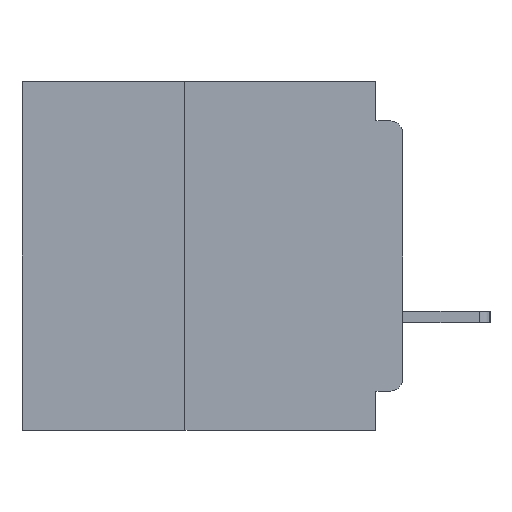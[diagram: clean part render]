
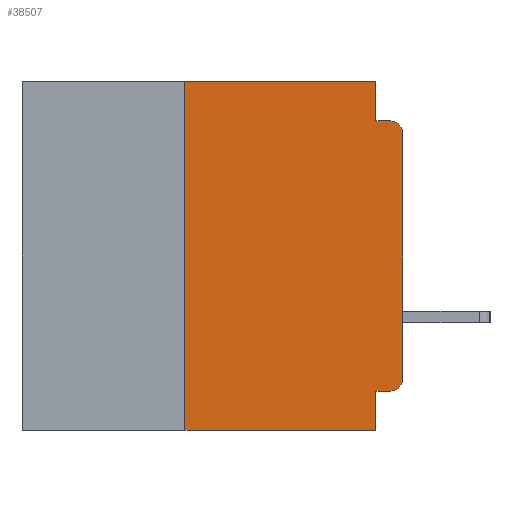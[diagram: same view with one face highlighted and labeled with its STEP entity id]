
A CAD part, left-side view. The second image highlights one B-rep face of the part: STEP entity #38507.
In plain terms, the highlighted planar face has unit normal (-1, 0, 0).
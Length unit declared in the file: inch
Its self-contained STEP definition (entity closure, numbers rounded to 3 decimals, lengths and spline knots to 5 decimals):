
#300 = EDGE_CURVE ( 'NONE', #31197, #36646, #64889, .T. ) ;
#389 = CARTESIAN_POINT ( 'NONE',  ( 0., 0.031, -0.355 ) ) ;
#638 = CARTESIAN_POINT ( 'NONE',  ( 0., 0., -0.06 ) ) ;
#1418 = ORIENTED_EDGE ( 'NONE', *, *, #44566, .F. ) ;
#1502 = DIRECTION ( 'NONE',  ( 0., 0., -1. ) ) ;
#1721 = AXIS2_PLACEMENT_3D ( 'NONE', #28137, #63955, #33288 ) ;
#1724 = EDGE_CURVE ( 'NONE', #13966, #51907, #29463, .T. ) ;
#1972 = CARTESIAN_POINT ( 'NONE',  ( 0., 0.437, 0. ) ) ;
#2990 = VERTEX_POINT ( 'NONE', #50784 ) ;
#3612 = VECTOR ( 'NONE', #39474, 39.37008 ) ;
#4235 = VERTEX_POINT ( 'NONE', #389 ) ;
#4448 = VECTOR ( 'NONE', #34540, 39.37008 ) ;
#4666 = LINE ( 'NONE', #46689, #44174 ) ;
#4717 = CARTESIAN_POINT ( 'NONE',  ( 0., 0.015, -0.045 ) ) ;
#6068 = ORIENTED_EDGE ( 'NONE', *, *, #1724, .T. ) ;
#6707 = LINE ( 'NONE', #27226, #58166 ) ;
#7853 = DIRECTION ( 'NONE',  ( 0., 0., -1. ) ) ;
#7986 = DIRECTION ( 'NONE',  ( -1., 0., 0. ) ) ;
#8141 = CARTESIAN_POINT ( 'NONE',  ( 0., 0.015, -0.06 ) ) ;
#8779 = EDGE_CURVE ( 'NONE', #31197, #39719, #44422, .T. ) ;
#9696 = CARTESIAN_POINT ( 'NONE',  ( 0., 0.437, 0. ) ) ;
#10513 = CIRCLE ( 'NONE', #1721, 0.015 ) ;
#12424 = EDGE_CURVE ( 'NONE', #45989, #31343, #10513, .T. ) ;
#13966 = VERTEX_POINT ( 'NONE', #638 ) ;
#14341 = ORIENTED_EDGE ( 'NONE', *, *, #63527, .F. ) ;
#16952 = VECTOR ( 'NONE', #34377, 39.37008 ) ;
#17418 = LINE ( 'NONE', #18843, #3612 ) ;
#18843 = CARTESIAN_POINT ( 'NONE',  ( 0., 0., -0.355 ) ) ;
#19035 = VECTOR ( 'NONE', #40504, 39.37008 ) ;
#20340 = EDGE_CURVE ( 'NONE', #31343, #13966, #59463, .T. ) ;
#21923 = FACE_OUTER_BOUND ( 'NONE', #22598, .T. ) ;
#22155 = ORIENTED_EDGE ( 'NONE', *, *, #12424, .T. ) ;
#22598 = EDGE_LOOP ( 'NONE', ( #47404, #6068, #56346, #14341, #60851, #65360, #43607, #38839, #1418, #22155 ) ) ;
#22989 = DIRECTION ( 'NONE',  ( 1., 0., 0. ) ) ;
#24036 = VECTOR ( 'NONE', #61606, 39.37008 ) ;
#24302 = EDGE_CURVE ( 'NONE', #36646, #2990, #32620, .T. ) ;
#26323 = CARTESIAN_POINT ( 'NONE',  ( 0., 0.015, -0.355 ) ) ;
#27226 = CARTESIAN_POINT ( 'NONE',  ( 0., 0.031, -0.4 ) ) ;
#28137 = CARTESIAN_POINT ( 'NONE',  ( 0., 0.015, -0.34 ) ) ;
#28972 = CARTESIAN_POINT ( 'NONE',  ( 0., 0.031, -0.4 ) ) ;
#29415 = CARTESIAN_POINT ( 'NONE',  ( 0., 0., -0.34 ) ) ;
#29463 = CIRCLE ( 'NONE', #58442, 0.015 ) ;
#30747 = VECTOR ( 'NONE', #58452, 39.37008 ) ;
#31197 = VERTEX_POINT ( 'NONE', #63880 ) ;
#31343 = VERTEX_POINT ( 'NONE', #29415 ) ;
#32190 = CARTESIAN_POINT ( 'NONE',  ( 0., 0.25, 0. ) ) ;
#32620 = LINE ( 'NONE', #9696, #19035 ) ;
#33288 = DIRECTION ( 'NONE',  ( 0., 0., -1. ) ) ;
#34369 = EDGE_CURVE ( 'NONE', #4235, #39719, #6707, .T. ) ;
#34377 = DIRECTION ( 'NONE',  ( 0., 0., 1. ) ) ;
#34540 = DIRECTION ( 'NONE',  ( 0., 0., -1. ) ) ;
#36646 = VERTEX_POINT ( 'NONE', #32190 ) ;
#38507 = ADVANCED_FACE ( 'NONE', ( #21923 ), #63750, .F. ) ;
#38839 = ORIENTED_EDGE ( 'NONE', *, *, #34369, .F. ) ;
#39474 = DIRECTION ( 'NONE',  ( 0., 1., 0. ) ) ;
#39719 = VERTEX_POINT ( 'NONE', #28972 ) ;
#39935 = VERTEX_POINT ( 'NONE', #56120 ) ;
#40504 = DIRECTION ( 'NONE',  ( 0., -1., 0. ) ) ;
#43607 = ORIENTED_EDGE ( 'NONE', *, *, #8779, .T. ) ;
#44174 = VECTOR ( 'NONE', #51844, 39.37008 ) ;
#44215 = AXIS2_PLACEMENT_3D ( 'NONE', #1972, #22989, #58860 ) ;
#44422 = LINE ( 'NONE', #48177, #30747 ) ;
#44566 = EDGE_CURVE ( 'NONE', #45989, #4235, #17418, .T. ) ;
#45989 = VERTEX_POINT ( 'NONE', #26323 ) ;
#46689 = CARTESIAN_POINT ( 'NONE',  ( 0., 0., -0.045 ) ) ;
#47404 = ORIENTED_EDGE ( 'NONE', *, *, #20340, .T. ) ;
#48177 = CARTESIAN_POINT ( 'NONE',  ( 0., 0.437, -0.4 ) ) ;
#49900 = EDGE_CURVE ( 'NONE', #39935, #51907, #4666, .T. ) ;
#50784 = CARTESIAN_POINT ( 'NONE',  ( 0., 0.031, 0. ) ) ;
#51844 = DIRECTION ( 'NONE',  ( 0., -1., 0. ) ) ;
#51907 = VERTEX_POINT ( 'NONE', #4717 ) ;
#56120 = CARTESIAN_POINT ( 'NONE',  ( 0., 0.031, -0.045 ) ) ;
#56346 = ORIENTED_EDGE ( 'NONE', *, *, #49900, .F. ) ;
#58166 = VECTOR ( 'NONE', #1502, 39.37008 ) ;
#58442 = AXIS2_PLACEMENT_3D ( 'NONE', #8141, #7986, #7853 ) ;
#58452 = DIRECTION ( 'NONE',  ( 0., -1., 0. ) ) ;
#58860 = DIRECTION ( 'NONE',  ( 0., 0., -1. ) ) ;
#59143 = LINE ( 'NONE', #60085, #4448 ) ;
#59463 = LINE ( 'NONE', #65010, #16952 ) ;
#60085 = CARTESIAN_POINT ( 'NONE',  ( 0., 0.031, 0. ) ) ;
#60851 = ORIENTED_EDGE ( 'NONE', *, *, #24302, .F. ) ;
#61606 = DIRECTION ( 'NONE',  ( 0., 0., 1. ) ) ;
#61674 = CARTESIAN_POINT ( 'NONE',  ( 0., 0.25, -0.4 ) ) ;
#63527 = EDGE_CURVE ( 'NONE', #2990, #39935, #59143, .T. ) ;
#63750 = PLANE ( 'NONE',  #44215 ) ;
#63880 = CARTESIAN_POINT ( 'NONE',  ( 0., 0.25, -0.4 ) ) ;
#63955 = DIRECTION ( 'NONE',  ( -1., 0., 0. ) ) ;
#64889 = LINE ( 'NONE', #61674, #24036 ) ;
#65010 = CARTESIAN_POINT ( 'NONE',  ( 0., 0., 0. ) ) ;
#65360 = ORIENTED_EDGE ( 'NONE', *, *, #300, .F. ) ;
